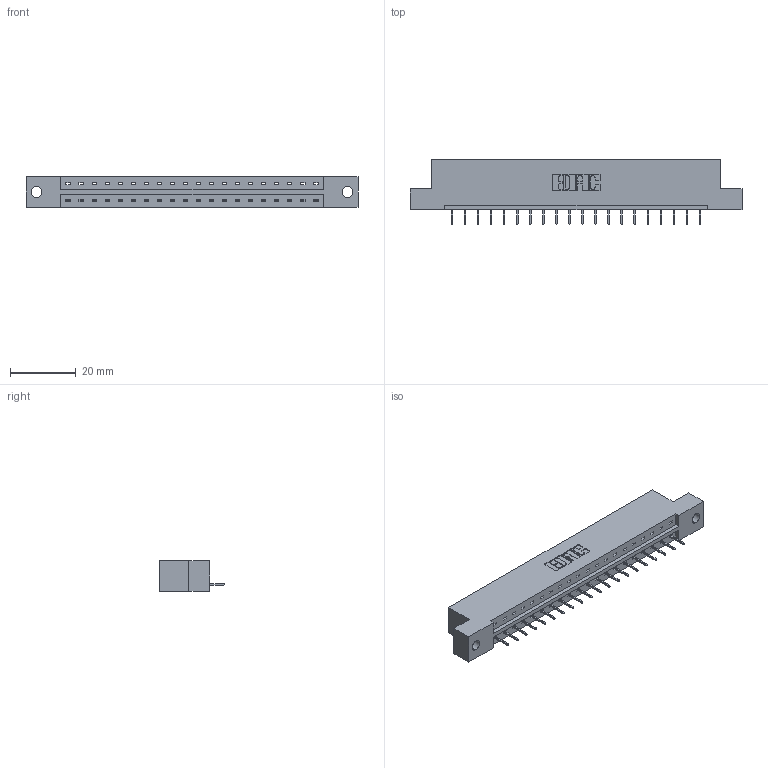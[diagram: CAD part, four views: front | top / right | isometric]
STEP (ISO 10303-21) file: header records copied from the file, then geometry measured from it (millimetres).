
FILE_DESCRIPTION (( 'STEP AP203' ), '1' );
FILE_NAME ('833-020-524-102.STEP', '2020-06-01T12:34:11', ( '' ), ( '' ), 'SwSTEP 2.0', 'SolidWorks 2020', '' );
FILE_SCHEMA (( 'CONFIG_CONTROL_DESIGN' ));
Length unit declared in the file: inch
Products named in the file (3): 833-020-524-102; 833 Part_Flush - .128 Dia; 345-292-001_345-293-124
Assembly tree (21 placements, depth 2):
  833-020-524-102
    833 Part_Flush - .128 Dia
    345-292-001_345-293-124  x20
Bounding box: 100.79 x 19.69 x 9.4 mm (x, y, z)
Volume: 9837.1 mm3; surface area: 9955.8 mm2
Topology: 21 solids, 21 shells, 1354 faces, 3911 edges, 2526 vertices
Faces by surface type: plane 1030, cylinder 324
Entity records: 15149 total; most frequent: CARTESIAN_POINT 2622, ORIENTED_EDGE 2578, DIRECTION 2257, EDGE_CURVE 1289, VECTOR 1165, LINE 1165, VERTEX_POINT 854, AXIS2_PLACEMENT_3D 546
